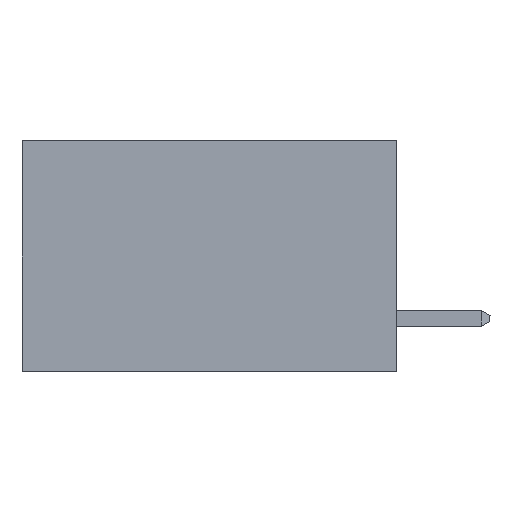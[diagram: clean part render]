
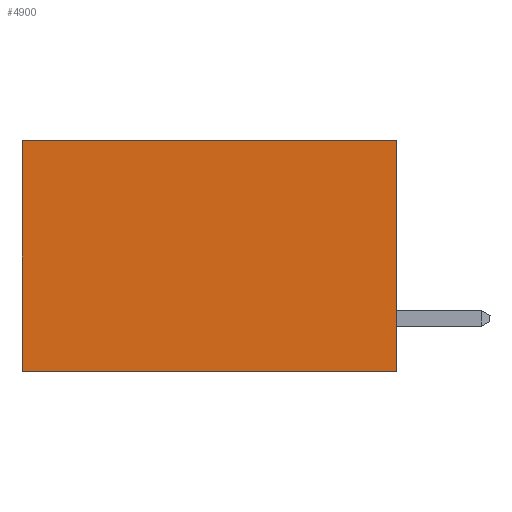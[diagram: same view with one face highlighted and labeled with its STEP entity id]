
A CAD part, left-side view. The second image highlights one B-rep face of the part: STEP entity #4900.
In plain terms, the highlighted planar face has unit normal (-1, 0, 0).
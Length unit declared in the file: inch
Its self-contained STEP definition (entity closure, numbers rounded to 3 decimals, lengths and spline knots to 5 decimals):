
#105 = ORIENTED_EDGE ( 'NONE', *, *, #3702, .T. ) ;
#590 = VERTEX_POINT ( 'NONE', #1563 ) ;
#597 = CARTESIAN_POINT ( 'NONE',  ( 0.2615, 0., -0.37 ) ) ;
#1003 = ORIENTED_EDGE ( 'NONE', *, *, #2180, .F. ) ;
#1164 = VERTEX_POINT ( 'NONE', #597 ) ;
#1167 = DIRECTION ( 'NONE',  ( 0., 0., -1. ) ) ;
#1233 = CARTESIAN_POINT ( 'NONE',  ( 0.2615, 0.6, -0.37 ) ) ;
#1451 = DIRECTION ( 'NONE',  ( 0., 1., 0. ) ) ;
#1563 = CARTESIAN_POINT ( 'NONE',  ( 0.2615, 0.6, -0.37 ) ) ;
#1992 = DIRECTION ( 'NONE',  ( 0., 1., 0. ) ) ;
#2083 = VECTOR ( 'NONE', #7405, 39.37008 ) ;
#2087 = VECTOR ( 'NONE', #1451, 39.37008 ) ;
#2180 = EDGE_CURVE ( 'NONE', #6634, #1164, #5072, .T. ) ;
#2371 = CARTESIAN_POINT ( 'NONE',  ( 0.2615, 0., 0. ) ) ;
#3552 = ORIENTED_EDGE ( 'NONE', *, *, #7795, .F. ) ;
#3702 = EDGE_CURVE ( 'NONE', #4642, #590, #6202, .T. ) ;
#4480 = DIRECTION ( 'NONE',  ( 0., 0., -1. ) ) ;
#4530 = DIRECTION ( 'NONE',  ( 1., 0., 0. ) ) ;
#4642 = VERTEX_POINT ( 'NONE', #10321 ) ;
#4668 = CARTESIAN_POINT ( 'NONE',  ( 0.2615, 0., -0.37 ) ) ;
#4748 = PLANE ( 'NONE',  #4785 ) ;
#4753 = LINE ( 'NONE', #9043, #2087 ) ;
#4785 = AXIS2_PLACEMENT_3D ( 'NONE', #4668, #4530, #4480 ) ;
#4900 = ADVANCED_FACE ( 'NONE', ( #7059 ), #4748, .F. ) ;
#5072 = LINE ( 'NONE', #6019, #2083 ) ;
#5915 = LINE ( 'NONE', #6882, #10695 ) ;
#6019 = CARTESIAN_POINT ( 'NONE',  ( 0.2615, 0., -0.37 ) ) ;
#6202 = LINE ( 'NONE', #1233, #10454 ) ;
#6634 = VERTEX_POINT ( 'NONE', #2371 ) ;
#6882 = CARTESIAN_POINT ( 'NONE',  ( 0.2615, 0., 0. ) ) ;
#7059 = FACE_OUTER_BOUND ( 'NONE', #11322, .T. ) ;
#7405 = DIRECTION ( 'NONE',  ( 0., 0., -1. ) ) ;
#7795 = EDGE_CURVE ( 'NONE', #1164, #590, #4753, .T. ) ;
#9043 = CARTESIAN_POINT ( 'NONE',  ( 0.2615, 0., -0.37 ) ) ;
#9336 = ORIENTED_EDGE ( 'NONE', *, *, #11266, .T. ) ;
#10321 = CARTESIAN_POINT ( 'NONE',  ( 0.2615, 0.6, 0. ) ) ;
#10454 = VECTOR ( 'NONE', #1167, 39.37008 ) ;
#10695 = VECTOR ( 'NONE', #1992, 39.37008 ) ;
#11266 = EDGE_CURVE ( 'NONE', #6634, #4642, #5915, .T. ) ;
#11322 = EDGE_LOOP ( 'NONE', ( #105, #3552, #1003, #9336 ) ) ;
